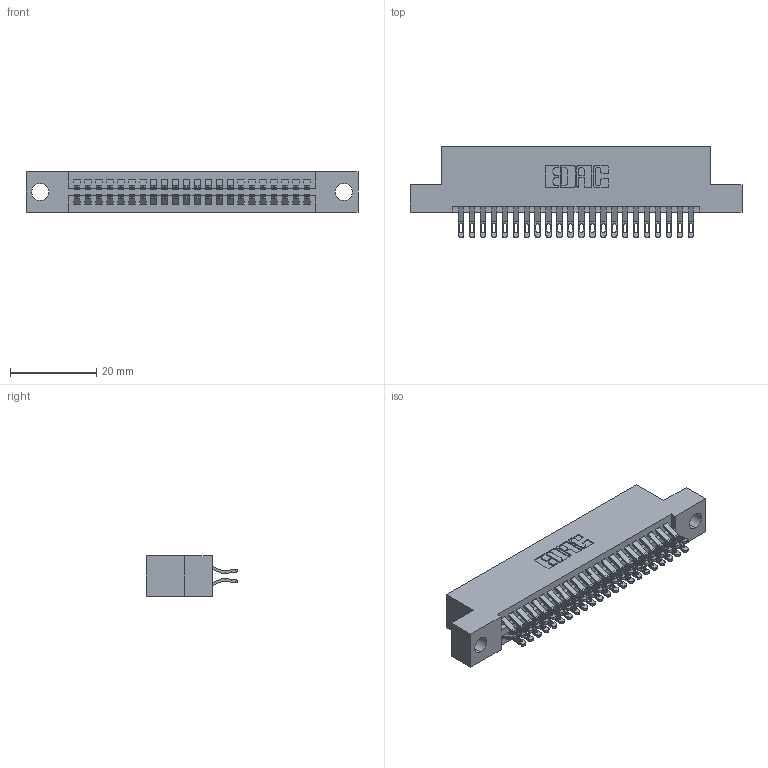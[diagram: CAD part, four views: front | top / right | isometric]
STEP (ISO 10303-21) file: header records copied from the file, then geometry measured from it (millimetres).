
FILE_DESCRIPTION (( 'STEP AP203' ), '1' );
FILE_NAME ('345-044-555-204.STEP', '2021-05-20T02:03:01', ( '' ), ( '' ), 'SwSTEP 2.0', 'SolidWorks 2020', '' );
FILE_SCHEMA (( 'CONFIG_CONTROL_DESIGN' ));
Length unit declared in the file: inch
Products named in the file (3): 345 Part_Flush Mounting Lugs - 0.156 Dia-TI; 345-044-555-204; 345-292-001_555 Tail
Assembly tree (45 placements, depth 2):
  345-044-555-204
    345 Part_Flush Mounting Lugs - 0.156 Dia-TI
    345-292-001_555 Tail  x44
Bounding box: 77.09 x 21.13 x 9.4 mm (x, y, z)
Volume: 7324.5 mm3; surface area: 10735 mm2
Topology: 45 solids, 45 shells, 2604 faces, 8165 edges, 5442 vertices
Faces by surface type: plane 1458, cylinder 1146
Entity records: 20699 total; most frequent: CARTESIAN_POINT 3528, ORIENTED_EDGE 3430, DIRECTION 3103, EDGE_CURVE 1715, VECTOR 1475, LINE 1475, VERTEX_POINT 1142, AXIS2_PLACEMENT_3D 814
